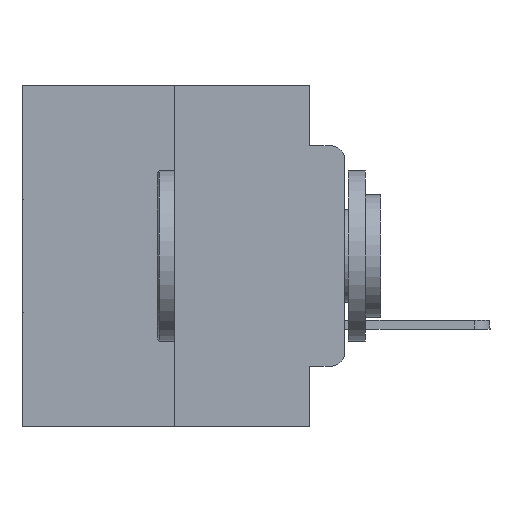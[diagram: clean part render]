
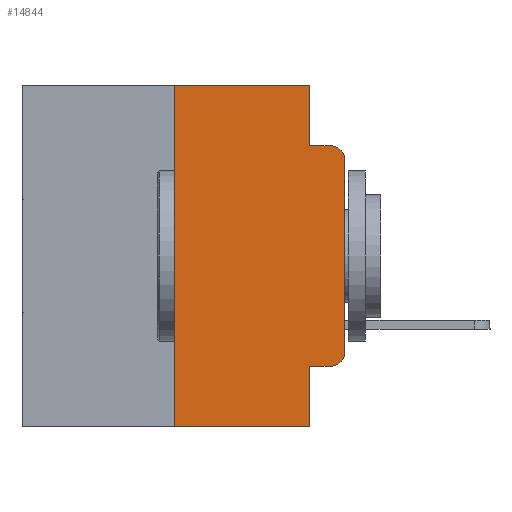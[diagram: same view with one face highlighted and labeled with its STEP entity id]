
A CAD part, left-side view. The second image highlights one B-rep face of the part: STEP entity #14844.
In plain terms, the highlighted planar face has unit normal (-1, 0, 0).
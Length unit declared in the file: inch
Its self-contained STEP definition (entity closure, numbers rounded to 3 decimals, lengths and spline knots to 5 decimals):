
#14 = CARTESIAN_POINT ( 'NONE',  ( 0., 0.051, -0.5 ) ) ;
#229 = CARTESIAN_POINT ( 'NONE',  ( 0., 0.25, 0. ) ) ;
#247 = PLANE ( 'NONE',  #9848 ) ;
#761 = EDGE_CURVE ( 'NONE', #8931, #24545, #25775, .T. ) ;
#1102 = AXIS2_PLACEMENT_3D ( 'NONE', #4013, #26015, #25452 ) ;
#1444 = DIRECTION ( 'NONE',  ( 0., -1., 0. ) ) ;
#1691 = CARTESIAN_POINT ( 'NONE',  ( 0., 0.051, -0.4115 ) ) ;
#2241 = DIRECTION ( 'NONE',  ( 0., -1., 0. ) ) ;
#3450 = CARTESIAN_POINT ( 'NONE',  ( 0., 0.02, -0.3915 ) ) ;
#4013 = CARTESIAN_POINT ( 'NONE',  ( 0., 0.02, -0.1085 ) ) ;
#4457 = CARTESIAN_POINT ( 'NONE',  ( 0., 0.051, 0. ) ) ;
#4515 = LINE ( 'NONE', #229, #5549 ) ;
#5549 = VECTOR ( 'NONE', #15696, 39.37008 ) ;
#5684 = AXIS2_PLACEMENT_3D ( 'NONE', #3450, #12184, #10157 ) ;
#5859 = EDGE_CURVE ( 'NONE', #24632, #21710, #7453, .T. ) ;
#5977 = VERTEX_POINT ( 'NONE', #26793 ) ;
#6066 = VERTEX_POINT ( 'NONE', #15651 ) ;
#6379 = DIRECTION ( 'NONE',  ( 0., -1., 0. ) ) ;
#6490 = VECTOR ( 'NONE', #6379, 39.37008 ) ;
#6913 = CARTESIAN_POINT ( 'NONE',  ( 0., 0., -0.1085 ) ) ;
#6942 = CARTESIAN_POINT ( 'NONE',  ( 0., 0.25, -0.5 ) ) ;
#7453 = LINE ( 'NONE', #20292, #19691 ) ;
#7976 = CIRCLE ( 'NONE', #5684, 0.02 ) ;
#8191 = ORIENTED_EDGE ( 'NONE', *, *, #14884, .T. ) ;
#8528 = CARTESIAN_POINT ( 'NONE',  ( 0., 0.473, 0. ) ) ;
#8627 = EDGE_CURVE ( 'NONE', #18202, #6066, #4515, .T. ) ;
#8665 = LINE ( 'NONE', #8528, #6490 ) ;
#8931 = VERTEX_POINT ( 'NONE', #14055 ) ;
#9450 = DIRECTION ( 'NONE',  ( 0., 0., -1. ) ) ;
#9666 = DIRECTION ( 'NONE',  ( 1., 0., 0. ) ) ;
#9848 = AXIS2_PLACEMENT_3D ( 'NONE', #11812, #9666, #17552 ) ;
#10157 = DIRECTION ( 'NONE',  ( 0., 0., -1. ) ) ;
#10210 = CARTESIAN_POINT ( 'NONE',  ( 0., 0.051, 0. ) ) ;
#10322 = CARTESIAN_POINT ( 'NONE',  ( 0., 0.051, -0.0885 ) ) ;
#10830 = CARTESIAN_POINT ( 'NONE',  ( 0., 0., 0. ) ) ;
#11259 = EDGE_CURVE ( 'NONE', #12698, #16129, #7976, .T. ) ;
#11812 = CARTESIAN_POINT ( 'NONE',  ( 0., 0.473, 0. ) ) ;
#12184 = DIRECTION ( 'NONE',  ( -1., 0., 0. ) ) ;
#12328 = LINE ( 'NONE', #10322, #17981 ) ;
#12650 = DIRECTION ( 'NONE',  ( 0., 0., -1. ) ) ;
#12698 = VERTEX_POINT ( 'NONE', #18445 ) ;
#13498 = VECTOR ( 'NONE', #2241, 39.37008 ) ;
#13704 = EDGE_CURVE ( 'NONE', #21710, #5977, #12328, .T. ) ;
#14055 = CARTESIAN_POINT ( 'NONE',  ( 0., 0.051, -0.4115 ) ) ;
#14844 = ADVANCED_FACE ( 'NONE', ( #15715 ), #247, .F. ) ;
#14884 = EDGE_CURVE ( 'NONE', #18202, #24545, #19835, .T. ) ;
#15199 = VERTEX_POINT ( 'NONE', #6913 ) ;
#15651 = CARTESIAN_POINT ( 'NONE',  ( 0., 0.25, 0. ) ) ;
#15696 = DIRECTION ( 'NONE',  ( 0., 0., 1. ) ) ;
#15715 = FACE_OUTER_BOUND ( 'NONE', #26731, .T. ) ;
#16006 = CARTESIAN_POINT ( 'NONE',  ( 0., 0., -0.3915 ) ) ;
#16129 = VERTEX_POINT ( 'NONE', #16006 ) ;
#16588 = CARTESIAN_POINT ( 'NONE',  ( 0., 0.051, -0.0885 ) ) ;
#17300 = EDGE_CURVE ( 'NONE', #8931, #12698, #21414, .T. ) ;
#17387 = DIRECTION ( 'NONE',  ( 0., 0., 1. ) ) ;
#17533 = ORIENTED_EDGE ( 'NONE', *, *, #13704, .F. ) ;
#17552 = DIRECTION ( 'NONE',  ( 0., 0., -1. ) ) ;
#17981 = VECTOR ( 'NONE', #1444, 39.37008 ) ;
#18202 = VERTEX_POINT ( 'NONE', #6942 ) ;
#18445 = CARTESIAN_POINT ( 'NONE',  ( 0., 0.02, -0.4115 ) ) ;
#19550 = DIRECTION ( 'NONE',  ( 0., -1., 0. ) ) ;
#19691 = VECTOR ( 'NONE', #9450, 39.37008 ) ;
#19835 = LINE ( 'NONE', #27214, #13498 ) ;
#20111 = EDGE_CURVE ( 'NONE', #15199, #5977, #23898, .T. ) ;
#20292 = CARTESIAN_POINT ( 'NONE',  ( 0., 0.051, 0. ) ) ;
#21396 = LINE ( 'NONE', #10830, #23713 ) ;
#21414 = LINE ( 'NONE', #1691, #27260 ) ;
#21660 = ORIENTED_EDGE ( 'NONE', *, *, #17300, .T. ) ;
#21710 = VERTEX_POINT ( 'NONE', #16588 ) ;
#21853 = VECTOR ( 'NONE', #12650, 39.37008 ) ;
#22567 = ORIENTED_EDGE ( 'NONE', *, *, #761, .F. ) ;
#23055 = ORIENTED_EDGE ( 'NONE', *, *, #11259, .T. ) ;
#23713 = VECTOR ( 'NONE', #17387, 39.37008 ) ;
#23898 = CIRCLE ( 'NONE', #1102, 0.02 ) ;
#24104 = EDGE_CURVE ( 'NONE', #16129, #15199, #21396, .T. ) ;
#24545 = VERTEX_POINT ( 'NONE', #14 ) ;
#24632 = VERTEX_POINT ( 'NONE', #4457 ) ;
#25452 = DIRECTION ( 'NONE',  ( 0., 0., -1. ) ) ;
#25775 = LINE ( 'NONE', #10210, #21853 ) ;
#26015 = DIRECTION ( 'NONE',  ( -1., 0., 0. ) ) ;
#26054 = ORIENTED_EDGE ( 'NONE', *, *, #27760, .F. ) ;
#26731 = EDGE_LOOP ( 'NONE', ( #26867, #28063, #17533, #27469, #26054, #28203, #8191, #22567, #21660, #23055 ) ) ;
#26793 = CARTESIAN_POINT ( 'NONE',  ( 0., 0.02, -0.0885 ) ) ;
#26867 = ORIENTED_EDGE ( 'NONE', *, *, #24104, .T. ) ;
#27214 = CARTESIAN_POINT ( 'NONE',  ( 0., 0.473, -0.5 ) ) ;
#27260 = VECTOR ( 'NONE', #19550, 39.37008 ) ;
#27469 = ORIENTED_EDGE ( 'NONE', *, *, #5859, .F. ) ;
#27760 = EDGE_CURVE ( 'NONE', #6066, #24632, #8665, .T. ) ;
#28063 = ORIENTED_EDGE ( 'NONE', *, *, #20111, .T. ) ;
#28203 = ORIENTED_EDGE ( 'NONE', *, *, #8627, .F. ) ;
